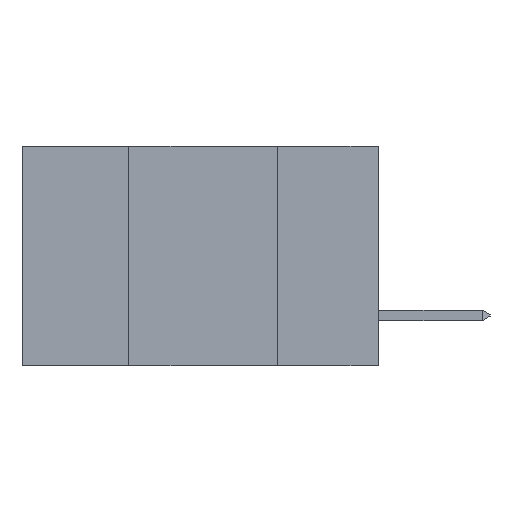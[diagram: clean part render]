
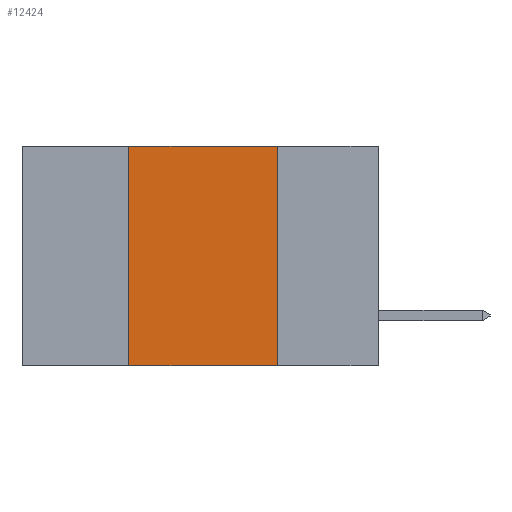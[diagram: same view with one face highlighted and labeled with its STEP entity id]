
A CAD part, left-side view. The second image highlights one B-rep face of the part: STEP entity #12424.
In plain terms, the highlighted planar face has unit normal (-1, 0, 0).
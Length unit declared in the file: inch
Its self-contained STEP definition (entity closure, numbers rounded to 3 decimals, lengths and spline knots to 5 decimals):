
#377 = EDGE_CURVE ( 'NONE', #917, #4982, #21186, .T. ) ;
#917 = VERTEX_POINT ( 'NONE', #4981 ) ;
#1458 = CARTESIAN_POINT ( 'NONE',  ( 0., 0.17, -0.37 ) ) ;
#1660 = ORIENTED_EDGE ( 'NONE', *, *, #377, .F. ) ;
#2498 = VECTOR ( 'NONE', #21187, 39.37008 ) ;
#2503 = VECTOR ( 'NONE', #21924, 39.37008 ) ;
#2820 = EDGE_CURVE ( 'NONE', #10754, #24180, #5218, .T. ) ;
#3049 = DIRECTION ( 'NONE',  ( 0., 0., -1. ) ) ;
#3702 = ORIENTED_EDGE ( 'NONE', *, *, #18365, .T. ) ;
#4368 = CARTESIAN_POINT ( 'NONE',  ( 0., 0.17, 0. ) ) ;
#4678 = CARTESIAN_POINT ( 'NONE',  ( 0., 0.17, -0.37 ) ) ;
#4981 = CARTESIAN_POINT ( 'NONE',  ( 0., 0.42, -0.37 ) ) ;
#4982 = VERTEX_POINT ( 'NONE', #17286 ) ;
#5218 = LINE ( 'NONE', #1458, #9120 ) ;
#5330 = ORIENTED_EDGE ( 'NONE', *, *, #23936, .F. ) ;
#6407 = AXIS2_PLACEMENT_3D ( 'NONE', #21487, #23388, #11890 ) ;
#7676 = LINE ( 'NONE', #14185, #2503 ) ;
#9120 = VECTOR ( 'NONE', #3049, 39.37008 ) ;
#9533 = ORIENTED_EDGE ( 'NONE', *, *, #2820, .F. ) ;
#9783 = DIRECTION ( 'NONE',  ( 0., 0., 1. ) ) ;
#9949 = PLANE ( 'NONE',  #6407 ) ;
#10754 = VERTEX_POINT ( 'NONE', #4368 ) ;
#10952 = VECTOR ( 'NONE', #9783, 39.37008 ) ;
#11890 = DIRECTION ( 'NONE',  ( 0., 0., -1. ) ) ;
#12200 = LINE ( 'NONE', #13537, #2498 ) ;
#12424 = ADVANCED_FACE ( 'NONE', ( #20376 ), #9949, .F. ) ;
#13537 = CARTESIAN_POINT ( 'NONE',  ( 0., 0.6, 0. ) ) ;
#14185 = CARTESIAN_POINT ( 'NONE',  ( 0., 0.6, -0.37 ) ) ;
#17286 = CARTESIAN_POINT ( 'NONE',  ( 0., 0.42, 0. ) ) ;
#17601 = EDGE_LOOP ( 'NONE', ( #9533, #5330, #1660, #3702 ) ) ;
#18365 = EDGE_CURVE ( 'NONE', #917, #24180, #7676, .T. ) ;
#20376 = FACE_OUTER_BOUND ( 'NONE', #17601, .T. ) ;
#20820 = CARTESIAN_POINT ( 'NONE',  ( 0., 0.42, -0.37 ) ) ;
#21186 = LINE ( 'NONE', #20820, #10952 ) ;
#21187 = DIRECTION ( 'NONE',  ( 0., -1., 0. ) ) ;
#21487 = CARTESIAN_POINT ( 'NONE',  ( 0., 0.6, 0. ) ) ;
#21924 = DIRECTION ( 'NONE',  ( 0., -1., 0. ) ) ;
#23388 = DIRECTION ( 'NONE',  ( 1., 0., 0. ) ) ;
#23936 = EDGE_CURVE ( 'NONE', #4982, #10754, #12200, .T. ) ;
#24180 = VERTEX_POINT ( 'NONE', #4678 ) ;
